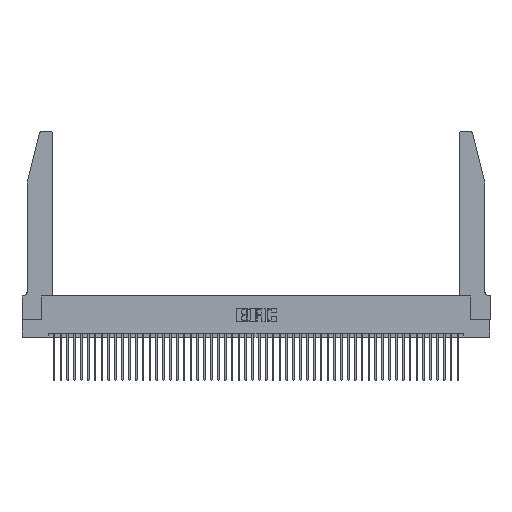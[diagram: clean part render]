
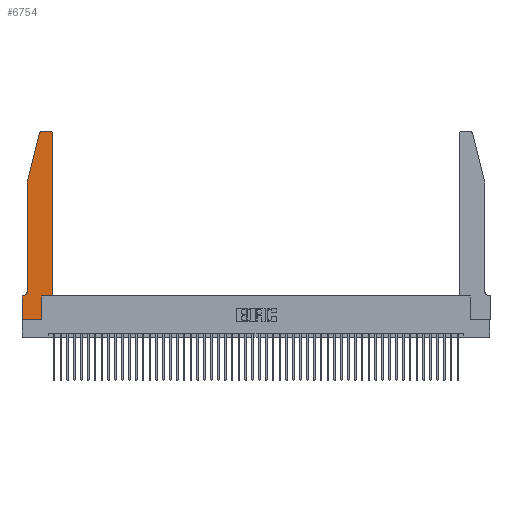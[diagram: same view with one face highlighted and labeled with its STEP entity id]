
A CAD part, top view. The second image highlights one B-rep face of the part: STEP entity #6754.
In plain terms, the highlighted planar face has unit normal (0, 0, 1).
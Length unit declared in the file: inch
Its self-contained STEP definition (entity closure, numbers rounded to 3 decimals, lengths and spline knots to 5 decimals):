
#102 = AXIS2_PLACEMENT_3D ( 'NONE', #14634, #6993, #26321 ) ;
#470 = PLANE ( 'NONE',  #7980 ) ;
#1201 = DIRECTION ( 'NONE',  ( -1., 0., 0. ) ) ;
#1527 = CARTESIAN_POINT ( 'NONE',  ( 0.4205, 2.72, 0.37 ) ) ;
#1541 = EDGE_CURVE ( 'NONE', #46960, #25986, #41260, .T. ) ;
#2327 = ORIENTED_EDGE ( 'NONE', *, *, #42951, .T. ) ;
#3558 = ORIENTED_EDGE ( 'NONE', *, *, #36366, .T. ) ;
#4297 = CARTESIAN_POINT ( 'NONE',  ( 0., 0.35, 0.37 ) ) ;
#4790 = CARTESIAN_POINT ( 'NONE',  ( 0.4205, 2.75, 0.37 ) ) ;
#4946 = EDGE_CURVE ( 'NONE', #32230, #26678, #29263, .T. ) ;
#5040 = CARTESIAN_POINT ( 'NONE',  ( 0.0755, 0.35, 0.37 ) ) ;
#5203 = CARTESIAN_POINT ( 'NONE',  ( 0.0755, 2., 0.37 ) ) ;
#5231 = DIRECTION ( 'NONE',  ( 0., 0., 1. ) ) ;
#5825 = DIRECTION ( 'NONE',  ( -0.239, -0.971, 0. ) ) ;
#5938 = ORIENTED_EDGE ( 'NONE', *, *, #47040, .T. ) ;
#6370 = DIRECTION ( 'NONE',  ( 0., -1., 0. ) ) ;
#6508 = CARTESIAN_POINT ( 'NONE',  ( 0.2605, 2.75, 0.37 ) ) ;
#6754 = ADVANCED_FACE ( 'NONE', ( #41619 ), #470, .T. ) ;
#6993 = DIRECTION ( 'NONE',  ( 0., 0., -1. ) ) ;
#6994 = LINE ( 'NONE', #6508, #31382 ) ;
#7276 = DIRECTION ( 'NONE',  ( 0., 0., 1. ) ) ;
#7312 = VECTOR ( 'NONE', #41631, 39.37008 ) ;
#7445 = CARTESIAN_POINT ( 'NONE',  ( 0.4505, 0.35, 0.37 ) ) ;
#7974 = LINE ( 'NONE', #15463, #13900 ) ;
#7980 = AXIS2_PLACEMENT_3D ( 'NONE', #4297, #45559, #22706 ) ;
#8698 = ORIENTED_EDGE ( 'NONE', *, *, #30579, .T. ) ;
#8719 = VECTOR ( 'NONE', #5825, 39.37008 ) ;
#9805 = DIRECTION ( 'NONE',  ( -1., 0., 0. ) ) ;
#10293 = LINE ( 'NONE', #5040, #25260 ) ;
#10469 = CARTESIAN_POINT ( 'NONE',  ( 0., 0.35, 0.37 ) ) ;
#12231 = EDGE_CURVE ( 'NONE', #17556, #46160, #22464, .T. ) ;
#13075 = VERTEX_POINT ( 'NONE', #44575 ) ;
#13539 = ORIENTED_EDGE ( 'NONE', *, *, #43548, .T. ) ;
#13900 = VECTOR ( 'NONE', #42189, 39.37008 ) ;
#14614 = DIRECTION ( 'NONE',  ( 0., -1., 0. ) ) ;
#14634 = CARTESIAN_POINT ( 'NONE',  ( 0.0055, 0.42, 0.37 ) ) ;
#15306 = CARTESIAN_POINT ( 'NONE',  ( 0.4505, 0.35, 0.37 ) ) ;
#15463 = CARTESIAN_POINT ( 'NONE',  ( 0.2865, 0.35, 0.37 ) ) ;
#16985 = CARTESIAN_POINT ( 'NONE',  ( 0.0755, 0.42, 0.37 ) ) ;
#17556 = VERTEX_POINT ( 'NONE', #45954 ) ;
#18612 = CARTESIAN_POINT ( 'NONE',  ( 0., 0., 0.37 ) ) ;
#18653 = EDGE_LOOP ( 'NONE', ( #47952, #31464, #5938, #2327, #30982, #3558, #13539, #8698, #31012, #32412, #37722, #24909 ) ) ;
#21407 = CARTESIAN_POINT ( 'NONE',  ( 0.0755, 2., 0.37 ) ) ;
#21725 = CARTESIAN_POINT ( 'NONE',  ( 0.4505, 0.35, 0.37 ) ) ;
#22249 = EDGE_CURVE ( 'NONE', #28703, #22463, #32761, .T. ) ;
#22463 = VERTEX_POINT ( 'NONE', #15306 ) ;
#22464 = CIRCLE ( 'NONE', #46139, 0.03 ) ;
#22706 = DIRECTION ( 'NONE',  ( 1., 0., 0. ) ) ;
#23002 = EDGE_CURVE ( 'NONE', #22463, #32230, #25518, .T. ) ;
#23677 = LINE ( 'NONE', #48527, #8719 ) ;
#24909 = ORIENTED_EDGE ( 'NONE', *, *, #4946, .T. ) ;
#25260 = VECTOR ( 'NONE', #1201, 39.37008 ) ;
#25518 = LINE ( 'NONE', #7445, #38080 ) ;
#25986 = VERTEX_POINT ( 'NONE', #34654 ) ;
#26321 = DIRECTION ( 'NONE',  ( -1., 0., 0. ) ) ;
#26678 = VERTEX_POINT ( 'NONE', #4790 ) ;
#27101 = CARTESIAN_POINT ( 'NONE',  ( 0.2865, 0.35, 0.37 ) ) ;
#27720 = CARTESIAN_POINT ( 'NONE',  ( 0.25487, 2.72718, 0.37 ) ) ;
#28703 = VERTEX_POINT ( 'NONE', #27101 ) ;
#29263 = CIRCLE ( 'NONE', #38296, 0.03 ) ;
#29802 = DIRECTION ( 'NONE',  ( 0., 1., 0. ) ) ;
#29973 = EDGE_CURVE ( 'NONE', #45765, #28703, #7974, .T. ) ;
#30100 = CARTESIAN_POINT ( 'NONE',  ( 0.284, 2.72, 0.37 ) ) ;
#30579 = EDGE_CURVE ( 'NONE', #13075, #45765, #37179, .T. ) ;
#30982 = ORIENTED_EDGE ( 'NONE', *, *, #1541, .T. ) ;
#31012 = ORIENTED_EDGE ( 'NONE', *, *, #29973, .T. ) ;
#31382 = VECTOR ( 'NONE', #9805, 39.37008 ) ;
#31464 = ORIENTED_EDGE ( 'NONE', *, *, #12231, .T. ) ;
#32230 = VERTEX_POINT ( 'NONE', #39686 ) ;
#32412 = ORIENTED_EDGE ( 'NONE', *, *, #22249, .T. ) ;
#32761 = LINE ( 'NONE', #21725, #41131 ) ;
#33007 = CARTESIAN_POINT ( 'NONE',  ( 0., 0., 0.37 ) ) ;
#34654 = CARTESIAN_POINT ( 'NONE',  ( 0.0055, 0.35, 0.37 ) ) ;
#36366 = EDGE_CURVE ( 'NONE', #25986, #39119, #10293, .T. ) ;
#36428 = DIRECTION ( 'NONE',  ( 1., 0., 0. ) ) ;
#37179 = LINE ( 'NONE', #18612, #7312 ) ;
#37722 = ORIENTED_EDGE ( 'NONE', *, *, #23002, .T. ) ;
#38080 = VECTOR ( 'NONE', #29802, 39.37008 ) ;
#38296 = AXIS2_PLACEMENT_3D ( 'NONE', #1527, #5231, #46804 ) ;
#39119 = VERTEX_POINT ( 'NONE', #10469 ) ;
#39686 = CARTESIAN_POINT ( 'NONE',  ( 0.4505, 2.72, 0.37 ) ) ;
#40170 = VECTOR ( 'NONE', #14614, 39.37008 ) ;
#40472 = EDGE_CURVE ( 'NONE', #26678, #17556, #6994, .T. ) ;
#40736 = LINE ( 'NONE', #33007, #40170 ) ;
#41131 = VECTOR ( 'NONE', #36428, 39.37008 ) ;
#41260 = CIRCLE ( 'NONE', #102, 0.07 ) ;
#41404 = LINE ( 'NONE', #21407, #42022 ) ;
#41619 = FACE_OUTER_BOUND ( 'NONE', #18653, .T. ) ;
#41631 = DIRECTION ( 'NONE',  ( 1., 0., 0. ) ) ;
#42022 = VECTOR ( 'NONE', #6370, 39.37008 ) ;
#42189 = DIRECTION ( 'NONE',  ( 0., 1., 0. ) ) ;
#42725 = VERTEX_POINT ( 'NONE', #5203 ) ;
#42951 = EDGE_CURVE ( 'NONE', #42725, #46960, #41404, .T. ) ;
#43548 = EDGE_CURVE ( 'NONE', #39119, #13075, #40736, .T. ) ;
#44575 = CARTESIAN_POINT ( 'NONE',  ( 0., 0., 0.37 ) ) ;
#45559 = DIRECTION ( 'NONE',  ( 0., 0., 1. ) ) ;
#45638 = DIRECTION ( 'NONE',  ( 1., 0., 0. ) ) ;
#45765 = VERTEX_POINT ( 'NONE', #47682 ) ;
#45954 = CARTESIAN_POINT ( 'NONE',  ( 0.284, 2.75, 0.37 ) ) ;
#46139 = AXIS2_PLACEMENT_3D ( 'NONE', #30100, #7276, #45638 ) ;
#46160 = VERTEX_POINT ( 'NONE', #27720 ) ;
#46804 = DIRECTION ( 'NONE',  ( 1., 0., 0. ) ) ;
#46960 = VERTEX_POINT ( 'NONE', #16985 ) ;
#47040 = EDGE_CURVE ( 'NONE', #46160, #42725, #23677, .T. ) ;
#47682 = CARTESIAN_POINT ( 'NONE',  ( 0.2865, 0., 0.37 ) ) ;
#47952 = ORIENTED_EDGE ( 'NONE', *, *, #40472, .T. ) ;
#48527 = CARTESIAN_POINT ( 'NONE',  ( 0.0755, 2., 0.37 ) ) ;
